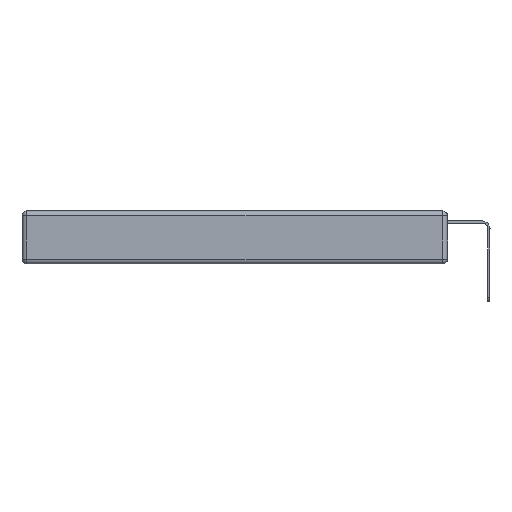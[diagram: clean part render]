
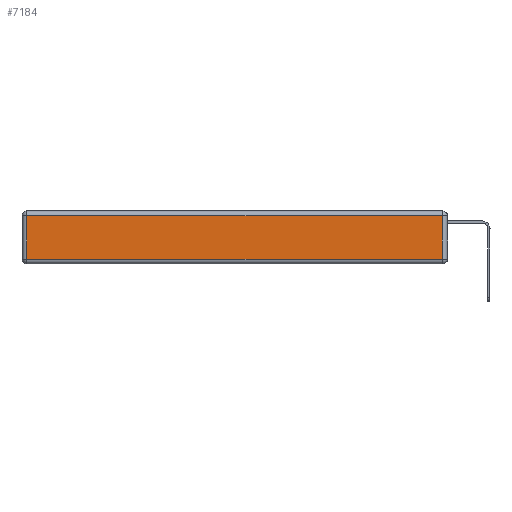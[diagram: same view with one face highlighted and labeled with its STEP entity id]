
A CAD part, left-side view. The second image highlights one B-rep face of the part: STEP entity #7184.
In plain terms, the highlighted planar face has unit normal (-1, 0, 0).
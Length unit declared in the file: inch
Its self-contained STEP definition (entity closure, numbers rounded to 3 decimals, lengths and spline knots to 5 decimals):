
#139 = VERTEX_POINT ( 'NONE', #9013 ) ;
#691 = CARTESIAN_POINT ( 'NONE',  ( 0., 0., -0.313 ) ) ;
#1461 = DIRECTION ( 'NONE',  ( 0., 0., 1. ) ) ;
#1832 = FACE_OUTER_BOUND ( 'NONE', #8414, .T. ) ;
#2038 = ORIENTED_EDGE ( 'NONE', *, *, #12801, .T. ) ;
#3245 = DIRECTION ( 'NONE',  ( 0., 0., 1. ) ) ;
#3427 = CARTESIAN_POINT ( 'NONE',  ( 0., 0., -0.343 ) ) ;
#3559 = DIRECTION ( 'NONE',  ( -1., 0., 0. ) ) ;
#3664 = ORIENTED_EDGE ( 'NONE', *, *, #7786, .T. ) ;
#4238 = VECTOR ( 'NONE', #3245, 39.37008 ) ;
#4463 = DIRECTION ( 'NONE',  ( 0., 1., 0. ) ) ;
#5324 = LINE ( 'NONE', #691, #6244 ) ;
#5608 = CARTESIAN_POINT ( 'NONE',  ( 0., 2.75, -0.03 ) ) ;
#5676 = AXIS2_PLACEMENT_3D ( 'NONE', #3427, #3559, #1461 ) ;
#6243 = EDGE_CURVE ( 'NONE', #9303, #10382, #7289, .T. ) ;
#6244 = VECTOR ( 'NONE', #6800, 39.37008 ) ;
#6292 = LINE ( 'NONE', #5608, #10573 ) ;
#6504 = PLANE ( 'NONE',  #5676 ) ;
#6739 = CARTESIAN_POINT ( 'NONE',  ( 0., 0.03, -0.313 ) ) ;
#6783 = ORIENTED_EDGE ( 'NONE', *, *, #6243, .T. ) ;
#6800 = DIRECTION ( 'NONE',  ( 0., -1., 0. ) ) ;
#7066 = CARTESIAN_POINT ( 'NONE',  ( 0., 2.72, -0.03 ) ) ;
#7184 = ADVANCED_FACE ( 'NONE', ( #1832 ), #6504, .T. ) ;
#7289 = LINE ( 'NONE', #8800, #9666 ) ;
#7786 = EDGE_CURVE ( 'NONE', #139, #9303, #6292, .T. ) ;
#7986 = VERTEX_POINT ( 'NONE', #6739 ) ;
#8035 = LINE ( 'NONE', #9347, #4238 ) ;
#8414 = EDGE_LOOP ( 'NONE', ( #2038, #8887, #3664, #6783 ) ) ;
#8800 = CARTESIAN_POINT ( 'NONE',  ( 0., 2.72, -0.343 ) ) ;
#8887 = ORIENTED_EDGE ( 'NONE', *, *, #8983, .T. ) ;
#8983 = EDGE_CURVE ( 'NONE', #7986, #139, #8035, .T. ) ;
#9013 = CARTESIAN_POINT ( 'NONE',  ( 0., 0.03, -0.03 ) ) ;
#9303 = VERTEX_POINT ( 'NONE', #7066 ) ;
#9347 = CARTESIAN_POINT ( 'NONE',  ( 0., 0.03, -0.343 ) ) ;
#9666 = VECTOR ( 'NONE', #12797, 39.37008 ) ;
#9922 = CARTESIAN_POINT ( 'NONE',  ( 0., 2.72, -0.313 ) ) ;
#10382 = VERTEX_POINT ( 'NONE', #9922 ) ;
#10573 = VECTOR ( 'NONE', #4463, 39.37008 ) ;
#12797 = DIRECTION ( 'NONE',  ( 0., 0., -1. ) ) ;
#12801 = EDGE_CURVE ( 'NONE', #10382, #7986, #5324, .T. ) ;
